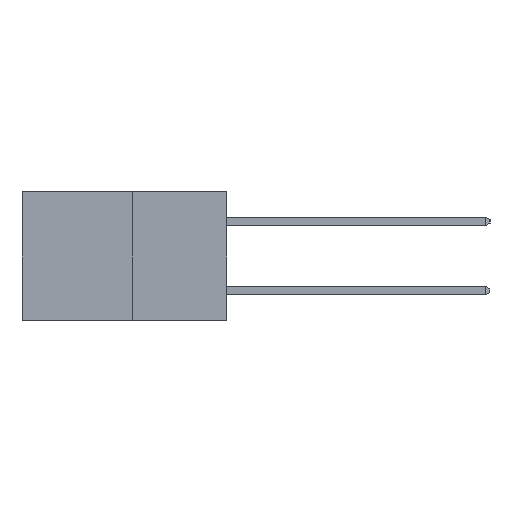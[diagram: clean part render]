
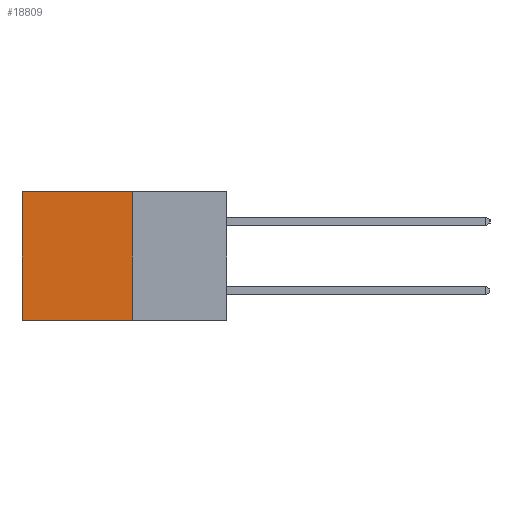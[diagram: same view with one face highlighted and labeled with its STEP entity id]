
A CAD part, left-side view. The second image highlights one B-rep face of the part: STEP entity #18809.
In plain terms, the highlighted planar face has unit normal (-1, 0, 0).
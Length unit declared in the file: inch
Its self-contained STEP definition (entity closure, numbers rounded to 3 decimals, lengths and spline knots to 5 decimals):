
#501 = ORIENTED_EDGE ( 'NONE', *, *, #15094, .T. ) ;
#732 = EDGE_LOOP ( 'NONE', ( #501, #6728, #17431, #5806 ) ) ;
#2094 = EDGE_CURVE ( 'NONE', #14728, #10020, #3086, .T. ) ;
#2809 = CARTESIAN_POINT ( 'NONE',  ( 0.277, 0.27, -0.37 ) ) ;
#3004 = LINE ( 'NONE', #16512, #11241 ) ;
#3086 = LINE ( 'NONE', #7088, #16379 ) ;
#3641 = CARTESIAN_POINT ( 'NONE',  ( 0.277, 0.59, -0.37 ) ) ;
#3768 = LINE ( 'NONE', #16660, #7899 ) ;
#4624 = DIRECTION ( 'NONE',  ( 0., 0., -1. ) ) ;
#5438 = DIRECTION ( 'NONE',  ( 0., 0., -1. ) ) ;
#5806 = ORIENTED_EDGE ( 'NONE', *, *, #2094, .T. ) ;
#6728 = ORIENTED_EDGE ( 'NONE', *, *, #20505, .F. ) ;
#7088 = CARTESIAN_POINT ( 'NONE',  ( 0.277, 0.27, 0. ) ) ;
#7516 = FACE_OUTER_BOUND ( 'NONE', #732, .T. ) ;
#7899 = VECTOR ( 'NONE', #8114, 39.37008 ) ;
#8114 = DIRECTION ( 'NONE',  ( 0., 0., -1. ) ) ;
#10020 = VERTEX_POINT ( 'NONE', #12969 ) ;
#10868 = LINE ( 'NONE', #3641, #19344 ) ;
#11241 = VECTOR ( 'NONE', #19899, 39.37008 ) ;
#11579 = PLANE ( 'NONE',  #18305 ) ;
#12969 = CARTESIAN_POINT ( 'NONE',  ( 0.277, 0.59, 0. ) ) ;
#13762 = CARTESIAN_POINT ( 'NONE',  ( 0.277, 0.27, -0.37 ) ) ;
#14728 = VERTEX_POINT ( 'NONE', #21559 ) ;
#14999 = DIRECTION ( 'NONE',  ( 1., 0., 0. ) ) ;
#15094 = EDGE_CURVE ( 'NONE', #10020, #22230, #10868, .T. ) ;
#16153 = EDGE_CURVE ( 'NONE', #14728, #19649, #3768, .T. ) ;
#16379 = VECTOR ( 'NONE', #19320, 39.37008 ) ;
#16512 = CARTESIAN_POINT ( 'NONE',  ( 0.277, 0.27, -0.37 ) ) ;
#16660 = CARTESIAN_POINT ( 'NONE',  ( 0.277, 0.27, -0.37 ) ) ;
#17431 = ORIENTED_EDGE ( 'NONE', *, *, #16153, .F. ) ;
#17797 = CARTESIAN_POINT ( 'NONE',  ( 0.277, 0.59, -0.37 ) ) ;
#18305 = AXIS2_PLACEMENT_3D ( 'NONE', #2809, #14999, #4624 ) ;
#18809 = ADVANCED_FACE ( 'NONE', ( #7516 ), #11579, .F. ) ;
#19320 = DIRECTION ( 'NONE',  ( 0., 1., 0. ) ) ;
#19344 = VECTOR ( 'NONE', #5438, 39.37008 ) ;
#19649 = VERTEX_POINT ( 'NONE', #13762 ) ;
#19899 = DIRECTION ( 'NONE',  ( 0., 1., 0. ) ) ;
#20505 = EDGE_CURVE ( 'NONE', #19649, #22230, #3004, .T. ) ;
#21559 = CARTESIAN_POINT ( 'NONE',  ( 0.277, 0.27, 0. ) ) ;
#22230 = VERTEX_POINT ( 'NONE', #17797 ) ;
